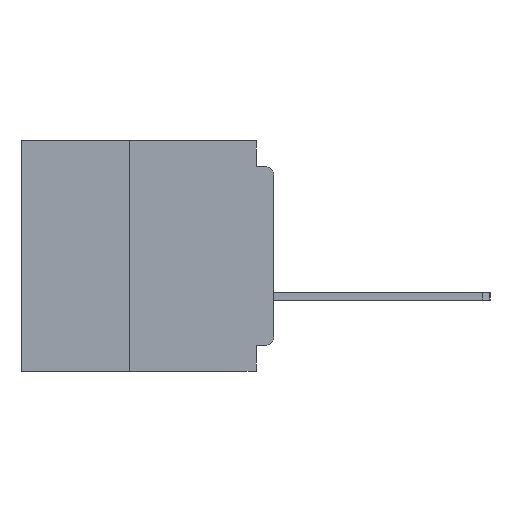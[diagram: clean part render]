
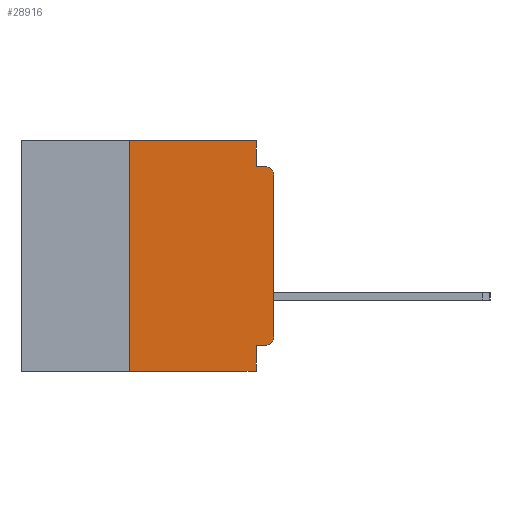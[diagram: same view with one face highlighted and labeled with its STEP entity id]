
A CAD part, left-side view. The second image highlights one B-rep face of the part: STEP entity #28916.
In plain terms, the highlighted planar face has unit normal (-1, 0, 0).
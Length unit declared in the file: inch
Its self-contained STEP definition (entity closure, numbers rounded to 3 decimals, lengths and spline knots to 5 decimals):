
#786 = DIRECTION ( 'NONE',  ( 0., 0., -1. ) ) ;
#986 = CARTESIAN_POINT ( 'NONE',  ( 0., 0.437, -0.4 ) ) ;
#1309 = CARTESIAN_POINT ( 'NONE',  ( 0., 0.25, -0.4 ) ) ;
#1557 = CARTESIAN_POINT ( 'NONE',  ( 0., 0.015, -0.355 ) ) ;
#1572 = LINE ( 'NONE', #7934, #12653 ) ;
#2888 = EDGE_CURVE ( 'NONE', #57636, #43992, #21741, .T. ) ;
#4584 = CARTESIAN_POINT ( 'NONE',  ( 0., 0., -0.045 ) ) ;
#5593 = DIRECTION ( 'NONE',  ( -1., 0., 0. ) ) ;
#5977 = AXIS2_PLACEMENT_3D ( 'NONE', #15169, #47383, #19802 ) ;
#6100 = ORIENTED_EDGE ( 'NONE', *, *, #16116, .F. ) ;
#7059 = VECTOR ( 'NONE', #29980, 39.37008 ) ;
#7382 = LINE ( 'NONE', #986, #41397 ) ;
#7934 = CARTESIAN_POINT ( 'NONE',  ( 0., 0., -0.355 ) ) ;
#9294 = DIRECTION ( 'NONE',  ( 0., -1., 0. ) ) ;
#9376 = EDGE_CURVE ( 'NONE', #45908, #25205, #29559, .T. ) ;
#9694 = CARTESIAN_POINT ( 'NONE',  ( 0., 0., -0.06 ) ) ;
#10027 = ORIENTED_EDGE ( 'NONE', *, *, #30030, .T. ) ;
#10450 = DIRECTION ( 'NONE',  ( 0., -1., 0. ) ) ;
#10669 = DIRECTION ( 'NONE',  ( 0., 0., -1. ) ) ;
#11992 = EDGE_CURVE ( 'NONE', #13453, #45908, #44338, .T. ) ;
#12640 = DIRECTION ( 'NONE',  ( 0., 1., 0. ) ) ;
#12653 = VECTOR ( 'NONE', #12640, 39.37008 ) ;
#13453 = VERTEX_POINT ( 'NONE', #28226 ) ;
#14712 = VECTOR ( 'NONE', #9294, 39.37008 ) ;
#15169 = CARTESIAN_POINT ( 'NONE',  ( 0., 0.015, -0.06 ) ) ;
#16116 = EDGE_CURVE ( 'NONE', #47845, #48586, #1572, .T. ) ;
#17464 = CARTESIAN_POINT ( 'NONE',  ( 0., 0.437, 0. ) ) ;
#19127 = AXIS2_PLACEMENT_3D ( 'NONE', #33418, #5593, #38020 ) ;
#19288 = VERTEX_POINT ( 'NONE', #55032 ) ;
#19439 = LINE ( 'NONE', #20661, #7059 ) ;
#19802 = DIRECTION ( 'NONE',  ( 0., 0., -1. ) ) ;
#20023 = AXIS2_PLACEMENT_3D ( 'NONE', #56285, #28766, #786 ) ;
#20168 = LINE ( 'NONE', #27865, #43266 ) ;
#20634 = ORIENTED_EDGE ( 'NONE', *, *, #11992, .F. ) ;
#20661 = CARTESIAN_POINT ( 'NONE',  ( 0., 0.25, -0.4 ) ) ;
#21200 = VERTEX_POINT ( 'NONE', #46443 ) ;
#21741 = CIRCLE ( 'NONE', #5977, 0.015 ) ;
#22762 = CARTESIAN_POINT ( 'NONE',  ( 0., 0.031, -0.4 ) ) ;
#25141 = EDGE_CURVE ( 'NONE', #48586, #19288, #26915, .T. ) ;
#25205 = VERTEX_POINT ( 'NONE', #50900 ) ;
#26915 = LINE ( 'NONE', #22762, #37697 ) ;
#27123 = ORIENTED_EDGE ( 'NONE', *, *, #27729, .T. ) ;
#27580 = EDGE_CURVE ( 'NONE', #25205, #43992, #51444, .T. ) ;
#27729 = EDGE_CURVE ( 'NONE', #29633, #19288, #7382, .T. ) ;
#27865 = CARTESIAN_POINT ( 'NONE',  ( 0., 0., 0. ) ) ;
#28226 = CARTESIAN_POINT ( 'NONE',  ( 0., 0.25, 0. ) ) ;
#28766 = DIRECTION ( 'NONE',  ( 1., 0., 0. ) ) ;
#28916 = ADVANCED_FACE ( 'NONE', ( #54892 ), #47027, .F. ) ;
#29174 = CARTESIAN_POINT ( 'NONE',  ( 0., 0.031, 0. ) ) ;
#29559 = LINE ( 'NONE', #29174, #52532 ) ;
#29633 = VERTEX_POINT ( 'NONE', #1309 ) ;
#29980 = DIRECTION ( 'NONE',  ( 0., 0., 1. ) ) ;
#30030 = EDGE_CURVE ( 'NONE', #21200, #57636, #20168, .T. ) ;
#32497 = DIRECTION ( 'NONE',  ( 0., 0., 1. ) ) ;
#33418 = CARTESIAN_POINT ( 'NONE',  ( 0., 0.015, -0.34 ) ) ;
#36089 = ORIENTED_EDGE ( 'NONE', *, *, #36454, .F. ) ;
#36292 = EDGE_CURVE ( 'NONE', #47845, #21200, #41842, .T. ) ;
#36435 = ORIENTED_EDGE ( 'NONE', *, *, #2888, .T. ) ;
#36454 = EDGE_CURVE ( 'NONE', #29633, #13453, #19439, .T. ) ;
#37697 = VECTOR ( 'NONE', #45895, 39.37008 ) ;
#38020 = DIRECTION ( 'NONE',  ( 0., 0., -1. ) ) ;
#41397 = VECTOR ( 'NONE', #10450, 39.37008 ) ;
#41842 = CIRCLE ( 'NONE', #19127, 0.015 ) ;
#42877 = VECTOR ( 'NONE', #49672, 39.37008 ) ;
#43266 = VECTOR ( 'NONE', #32497, 39.37008 ) ;
#43992 = VERTEX_POINT ( 'NONE', #48983 ) ;
#44338 = LINE ( 'NONE', #17464, #42877 ) ;
#45243 = CARTESIAN_POINT ( 'NONE',  ( 0., 0.031, 0. ) ) ;
#45895 = DIRECTION ( 'NONE',  ( 0., 0., -1. ) ) ;
#45908 = VERTEX_POINT ( 'NONE', #45243 ) ;
#46443 = CARTESIAN_POINT ( 'NONE',  ( 0., 0., -0.34 ) ) ;
#46555 = ORIENTED_EDGE ( 'NONE', *, *, #27580, .F. ) ;
#47027 = PLANE ( 'NONE',  #20023 ) ;
#47383 = DIRECTION ( 'NONE',  ( -1., 0., 0. ) ) ;
#47756 = EDGE_LOOP ( 'NONE', ( #10027, #36435, #46555, #55480, #20634, #36089, #27123, #50245, #6100, #55591 ) ) ;
#47845 = VERTEX_POINT ( 'NONE', #1557 ) ;
#48586 = VERTEX_POINT ( 'NONE', #49736 ) ;
#48983 = CARTESIAN_POINT ( 'NONE',  ( 0., 0.015, -0.045 ) ) ;
#49672 = DIRECTION ( 'NONE',  ( 0., -1., 0. ) ) ;
#49736 = CARTESIAN_POINT ( 'NONE',  ( 0., 0.031, -0.355 ) ) ;
#50245 = ORIENTED_EDGE ( 'NONE', *, *, #25141, .F. ) ;
#50900 = CARTESIAN_POINT ( 'NONE',  ( 0., 0.031, -0.045 ) ) ;
#51444 = LINE ( 'NONE', #4584, #14712 ) ;
#52532 = VECTOR ( 'NONE', #10669, 39.37008 ) ;
#54892 = FACE_OUTER_BOUND ( 'NONE', #47756, .T. ) ;
#55032 = CARTESIAN_POINT ( 'NONE',  ( 0., 0.031, -0.4 ) ) ;
#55480 = ORIENTED_EDGE ( 'NONE', *, *, #9376, .F. ) ;
#55591 = ORIENTED_EDGE ( 'NONE', *, *, #36292, .T. ) ;
#56285 = CARTESIAN_POINT ( 'NONE',  ( 0., 0.437, 0. ) ) ;
#57636 = VERTEX_POINT ( 'NONE', #9694 ) ;
